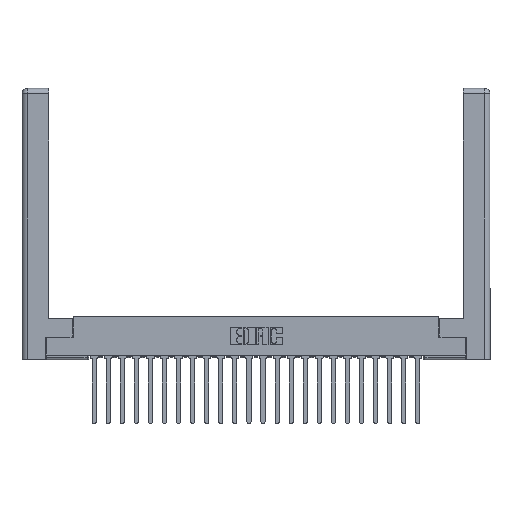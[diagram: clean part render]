
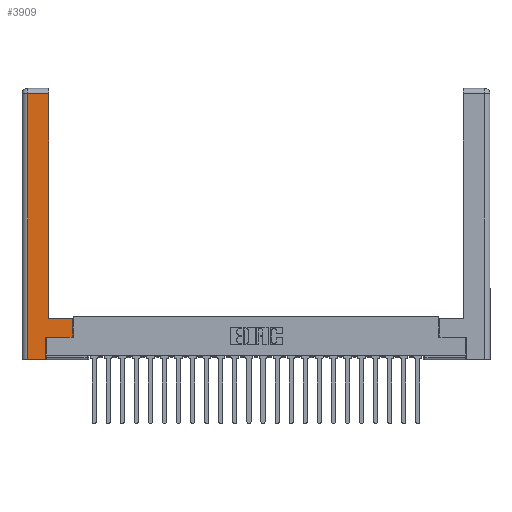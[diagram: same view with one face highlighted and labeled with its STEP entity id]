
A CAD part, top view. The second image highlights one B-rep face of the part: STEP entity #3909.
In plain terms, the highlighted planar face has unit normal (0, 0, 1).
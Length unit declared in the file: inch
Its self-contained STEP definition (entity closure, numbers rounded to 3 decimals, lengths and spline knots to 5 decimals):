
#71 = CARTESIAN_POINT ( 'NONE',  ( 0.565, 0.45, 0. ) ) ;
#609 = CARTESIAN_POINT ( 'NONE',  ( 0., 0., 0. ) ) ;
#866 = DIRECTION ( 'NONE',  ( -1., 0., 0. ) ) ;
#883 = CARTESIAN_POINT ( 'NONE',  ( 0.265, 0., 0. ) ) ;
#1197 = ORIENTED_EDGE ( 'NONE', *, *, #2271, .T. ) ;
#1331 = DIRECTION ( 'NONE',  ( 1., 0., 0. ) ) ;
#1828 = VECTOR ( 'NONE', #18219, 39.37008 ) ;
#2158 = EDGE_CURVE ( 'NONE', #8504, #16605, #12974, .T. ) ;
#2162 = EDGE_CURVE ( 'NONE', #7719, #8504, #5039, .T. ) ;
#2190 = VECTOR ( 'NONE', #20042, 39.37008 ) ;
#2271 = EDGE_CURVE ( 'NONE', #12842, #23734, #14576, .T. ) ;
#2297 = AXIS2_PLACEMENT_3D ( 'NONE', #609, #18923, #866 ) ;
#2582 = CARTESIAN_POINT ( 'NONE',  ( 0.265, 0.245, 0. ) ) ;
#3725 = FACE_OUTER_BOUND ( 'NONE', #20192, .T. ) ;
#3746 = ORIENTED_EDGE ( 'NONE', *, *, #7395, .T. ) ;
#3784 = ORIENTED_EDGE ( 'NONE', *, *, #2162, .T. ) ;
#3823 = ORIENTED_EDGE ( 'NONE', *, *, #24751, .T. ) ;
#3909 = ADVANCED_FACE ( 'NONE', ( #3725 ), #13009, .F. ) ;
#5039 = LINE ( 'NONE', #9890, #2190 ) ;
#5208 = CARTESIAN_POINT ( 'NONE',  ( 0.565, 0.245, 0. ) ) ;
#5987 = VECTOR ( 'NONE', #1331, 39.37008 ) ;
#6117 = CARTESIAN_POINT ( 'NONE',  ( 0.265, 0.245, 0. ) ) ;
#6465 = VECTOR ( 'NONE', #13111, 39.37008 ) ;
#6495 = VERTEX_POINT ( 'NONE', #12132 ) ;
#7104 = CARTESIAN_POINT ( 'NONE',  ( 0.0615, 2.94, 0. ) ) ;
#7182 = LINE ( 'NONE', #2582, #20494 ) ;
#7241 = ORIENTED_EDGE ( 'NONE', *, *, #16385, .T. ) ;
#7395 = EDGE_CURVE ( 'NONE', #6495, #21998, #20073, .T. ) ;
#7451 = ORIENTED_EDGE ( 'NONE', *, *, #23667, .T. ) ;
#7536 = CARTESIAN_POINT ( 'NONE',  ( 0.295, 0.45, 0. ) ) ;
#7719 = VERTEX_POINT ( 'NONE', #24314 ) ;
#8461 = VERTEX_POINT ( 'NONE', #20991 ) ;
#8504 = VERTEX_POINT ( 'NONE', #25135 ) ;
#8845 = VECTOR ( 'NONE', #19273, 39.37008 ) ;
#9890 = CARTESIAN_POINT ( 'NONE',  ( 0.295, 3., 0. ) ) ;
#11795 = DIRECTION ( 'NONE',  ( -1., 0., 0. ) ) ;
#11919 = CARTESIAN_POINT ( 'NONE',  ( 0.0615, 2.94, 0. ) ) ;
#12132 = CARTESIAN_POINT ( 'NONE',  ( 0.0615, 0., 0. ) ) ;
#12842 = VERTEX_POINT ( 'NONE', #6117 ) ;
#12974 = LINE ( 'NONE', #11919, #15855 ) ;
#13009 = PLANE ( 'NONE',  #2297 ) ;
#13111 = DIRECTION ( 'NONE',  ( 1., 0., 0. ) ) ;
#14576 = LINE ( 'NONE', #5208, #5987 ) ;
#14791 = ORIENTED_EDGE ( 'NONE', *, *, #2158, .T. ) ;
#15197 = LINE ( 'NONE', #17360, #8845 ) ;
#15855 = VECTOR ( 'NONE', #25794, 39.37008 ) ;
#16385 = EDGE_CURVE ( 'NONE', #23734, #8461, #21757, .T. ) ;
#16605 = VERTEX_POINT ( 'NONE', #7104 ) ;
#16701 = LINE ( 'NONE', #7536, #17340 ) ;
#17340 = VECTOR ( 'NONE', #11795, 39.37008 ) ;
#17360 = CARTESIAN_POINT ( 'NONE',  ( 0.0615, 0., 0. ) ) ;
#17632 = CARTESIAN_POINT ( 'NONE',  ( 0.565, 0.245, 0. ) ) ;
#17713 = CARTESIAN_POINT ( 'NONE',  ( 0.265, 0., 0. ) ) ;
#18219 = DIRECTION ( 'NONE',  ( 0., 1., 0. ) ) ;
#18923 = DIRECTION ( 'NONE',  ( 0., 0., -1. ) ) ;
#19273 = DIRECTION ( 'NONE',  ( 0., -1., 0. ) ) ;
#20042 = DIRECTION ( 'NONE',  ( 0., 1., 0. ) ) ;
#20073 = LINE ( 'NONE', #883, #6465 ) ;
#20192 = EDGE_LOOP ( 'NONE', ( #3784, #14791, #7451, #3746, #3823, #1197, #7241, #24342 ) ) ;
#20494 = VECTOR ( 'NONE', #22770, 39.37008 ) ;
#20991 = CARTESIAN_POINT ( 'NONE',  ( 0.565, 0.45, 0. ) ) ;
#21294 = EDGE_CURVE ( 'NONE', #8461, #7719, #16701, .T. ) ;
#21757 = LINE ( 'NONE', #71, #1828 ) ;
#21998 = VERTEX_POINT ( 'NONE', #17713 ) ;
#22770 = DIRECTION ( 'NONE',  ( 0., 1., 0. ) ) ;
#23667 = EDGE_CURVE ( 'NONE', #16605, #6495, #15197, .T. ) ;
#23734 = VERTEX_POINT ( 'NONE', #17632 ) ;
#24314 = CARTESIAN_POINT ( 'NONE',  ( 0.295, 0.45, 0. ) ) ;
#24342 = ORIENTED_EDGE ( 'NONE', *, *, #21294, .T. ) ;
#24751 = EDGE_CURVE ( 'NONE', #21998, #12842, #7182, .T. ) ;
#25135 = CARTESIAN_POINT ( 'NONE',  ( 0.295, 2.94, 0. ) ) ;
#25794 = DIRECTION ( 'NONE',  ( -1., 0., 0. ) ) ;
